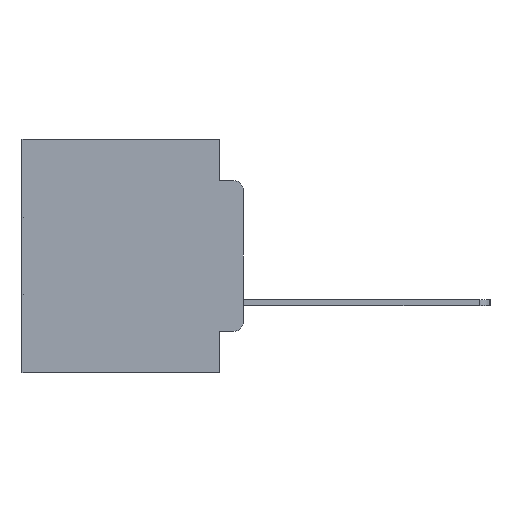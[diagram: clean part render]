
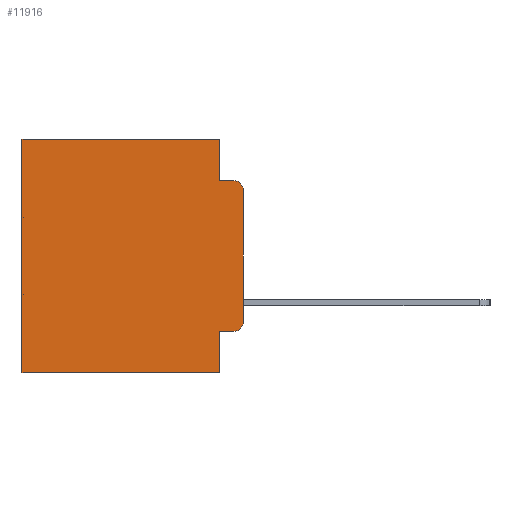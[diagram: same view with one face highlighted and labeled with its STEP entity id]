
A CAD part, left-side view. The second image highlights one B-rep face of the part: STEP entity #11916.
In plain terms, the highlighted planar face has unit normal (-1, 0, 0).
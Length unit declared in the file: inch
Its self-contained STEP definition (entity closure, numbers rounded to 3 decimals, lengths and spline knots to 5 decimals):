
#603 = DIRECTION ( 'NONE',  ( 0., -1., 0. ) ) ;
#1709 = EDGE_CURVE ( 'NONE', #10715, #7842, #5177, .T. ) ;
#1753 = VECTOR ( 'NONE', #17939, 39.37008 ) ;
#1819 = ORIENTED_EDGE ( 'NONE', *, *, #19235, .T. ) ;
#2353 = LINE ( 'NONE', #12784, #19906 ) ;
#3320 = ORIENTED_EDGE ( 'NONE', *, *, #22223, .F. ) ;
#3556 = DIRECTION ( 'NONE',  ( 0., 0., -1. ) ) ;
#3908 = VECTOR ( 'NONE', #603, 39.37008 ) ;
#3917 = VERTEX_POINT ( 'NONE', #16243 ) ;
#4325 = CARTESIAN_POINT ( 'NONE',  ( 0.298, 0., 0. ) ) ;
#4827 = CARTESIAN_POINT ( 'NONE',  ( 0.298, 0.02, -0.1085 ) ) ;
#5134 = ORIENTED_EDGE ( 'NONE', *, *, #26665, .T. ) ;
#5177 = LINE ( 'NONE', #9170, #16693 ) ;
#5872 = DIRECTION ( 'NONE',  ( 0., 1., 0. ) ) ;
#6313 = EDGE_CURVE ( 'NONE', #16755, #18127, #15384, .T. ) ;
#6566 = DIRECTION ( 'NONE',  ( 0., 0., -1. ) ) ;
#7085 = EDGE_CURVE ( 'NONE', #11197, #7842, #18121, .T. ) ;
#7178 = VERTEX_POINT ( 'NONE', #7598 ) ;
#7215 = DIRECTION ( 'NONE',  ( 0., 0., -1. ) ) ;
#7394 = CARTESIAN_POINT ( 'NONE',  ( 0.298, 0.02, -0.3915 ) ) ;
#7598 = CARTESIAN_POINT ( 'NONE',  ( 0.298, 0.051, -0.4115 ) ) ;
#7682 = LINE ( 'NONE', #4325, #24909 ) ;
#7842 = VERTEX_POINT ( 'NONE', #12554 ) ;
#8061 = LINE ( 'NONE', #13428, #1753 ) ;
#8157 = CARTESIAN_POINT ( 'NONE',  ( 0.298, 0., -0.5 ) ) ;
#8674 = LINE ( 'NONE', #16896, #3908 ) ;
#8847 = DIRECTION ( 'NONE',  ( 0., 0., -1. ) ) ;
#9170 = CARTESIAN_POINT ( 'NONE',  ( 0.298, 0., 0. ) ) ;
#9320 = VECTOR ( 'NONE', #5872, 39.37008 ) ;
#9336 = DIRECTION ( 'NONE',  ( 0., 0., -1. ) ) ;
#9675 = AXIS2_PLACEMENT_3D ( 'NONE', #20094, #22314, #8847 ) ;
#9716 = VERTEX_POINT ( 'NONE', #14064 ) ;
#9718 = DIRECTION ( 'NONE',  ( 0., 0., -1. ) ) ;
#9772 = VERTEX_POINT ( 'NONE', #25300 ) ;
#9780 = LINE ( 'NONE', #22777, #21048 ) ;
#10213 = EDGE_CURVE ( 'NONE', #9716, #3917, #7682, .T. ) ;
#10715 = VERTEX_POINT ( 'NONE', #26835 ) ;
#10894 = DIRECTION ( 'NONE',  ( 0., 0., -1. ) ) ;
#10975 = ORIENTED_EDGE ( 'NONE', *, *, #6313, .F. ) ;
#11088 = CARTESIAN_POINT ( 'NONE',  ( 0.298, 0.051, -0.5 ) ) ;
#11197 = VERTEX_POINT ( 'NONE', #12771 ) ;
#11686 = EDGE_CURVE ( 'NONE', #7178, #11197, #8674, .T. ) ;
#11916 = ADVANCED_FACE ( 'NONE', ( #18911 ), #17864, .F. ) ;
#12554 = CARTESIAN_POINT ( 'NONE',  ( 0.298, 0., -0.3915 ) ) ;
#12771 = CARTESIAN_POINT ( 'NONE',  ( 0.298, 0.02, -0.4115 ) ) ;
#12784 = CARTESIAN_POINT ( 'NONE',  ( 0.298, 0.051, 0. ) ) ;
#13408 = CARTESIAN_POINT ( 'NONE',  ( 0.298, 0.473, 0. ) ) ;
#13428 = CARTESIAN_POINT ( 'NONE',  ( 0.298, 0.051, -0.0885 ) ) ;
#13440 = CARTESIAN_POINT ( 'NONE',  ( 0.298, 0.473, -0.5 ) ) ;
#13480 = CIRCLE ( 'NONE', #25798, 0.02 ) ;
#13502 = ORIENTED_EDGE ( 'NONE', *, *, #10213, .T. ) ;
#13549 = DIRECTION ( 'NONE',  ( 0., 1., 0. ) ) ;
#13873 = ORIENTED_EDGE ( 'NONE', *, *, #11686, .T. ) ;
#14064 = CARTESIAN_POINT ( 'NONE',  ( 0.298, 0.051, 0. ) ) ;
#14256 = EDGE_LOOP ( 'NONE', ( #15628, #5134, #23213, #3320, #13502, #1819, #10975, #20507, #13873, #15281 ) ) ;
#14568 = CARTESIAN_POINT ( 'NONE',  ( 0.298, 0.02, -0.0885 ) ) ;
#14606 = VECTOR ( 'NONE', #6566, 39.37008 ) ;
#15281 = ORIENTED_EDGE ( 'NONE', *, *, #7085, .T. ) ;
#15384 = LINE ( 'NONE', #8157, #9320 ) ;
#15628 = ORIENTED_EDGE ( 'NONE', *, *, #1709, .F. ) ;
#16243 = CARTESIAN_POINT ( 'NONE',  ( 0.298, 0.473, 0. ) ) ;
#16273 = EDGE_CURVE ( 'NONE', #7178, #16755, #9780, .T. ) ;
#16693 = VECTOR ( 'NONE', #10894, 39.37008 ) ;
#16755 = VERTEX_POINT ( 'NONE', #11088 ) ;
#16896 = CARTESIAN_POINT ( 'NONE',  ( 0.298, 0.051, -0.4115 ) ) ;
#17864 = PLANE ( 'NONE',  #9675 ) ;
#17939 = DIRECTION ( 'NONE',  ( 0., -1., 0. ) ) ;
#18121 = CIRCLE ( 'NONE', #22732, 0.02 ) ;
#18127 = VERTEX_POINT ( 'NONE', #13440 ) ;
#18911 = FACE_OUTER_BOUND ( 'NONE', #14256, .T. ) ;
#19235 = EDGE_CURVE ( 'NONE', #3917, #18127, #27112, .T. ) ;
#19906 = VECTOR ( 'NONE', #3556, 39.37008 ) ;
#20094 = CARTESIAN_POINT ( 'NONE',  ( 0.298, 0., 0. ) ) ;
#20507 = ORIENTED_EDGE ( 'NONE', *, *, #16273, .F. ) ;
#20767 = DIRECTION ( 'NONE',  ( -1., 0., 0. ) ) ;
#21048 = VECTOR ( 'NONE', #9336, 39.37008 ) ;
#22223 = EDGE_CURVE ( 'NONE', #9716, #9772, #2353, .T. ) ;
#22314 = DIRECTION ( 'NONE',  ( 1., 0., 0. ) ) ;
#22732 = AXIS2_PLACEMENT_3D ( 'NONE', #7394, #23135, #9718 ) ;
#22755 = VERTEX_POINT ( 'NONE', #14568 ) ;
#22777 = CARTESIAN_POINT ( 'NONE',  ( 0.298, 0.051, 0. ) ) ;
#23135 = DIRECTION ( 'NONE',  ( -1., 0., 0. ) ) ;
#23213 = ORIENTED_EDGE ( 'NONE', *, *, #25158, .F. ) ;
#24909 = VECTOR ( 'NONE', #13549, 39.37008 ) ;
#25158 = EDGE_CURVE ( 'NONE', #9772, #22755, #8061, .T. ) ;
#25300 = CARTESIAN_POINT ( 'NONE',  ( 0.298, 0.051, -0.0885 ) ) ;
#25798 = AXIS2_PLACEMENT_3D ( 'NONE', #4827, #20767, #7215 ) ;
#26665 = EDGE_CURVE ( 'NONE', #10715, #22755, #13480, .T. ) ;
#26835 = CARTESIAN_POINT ( 'NONE',  ( 0.298, 0., -0.1085 ) ) ;
#27112 = LINE ( 'NONE', #13408, #14606 ) ;
